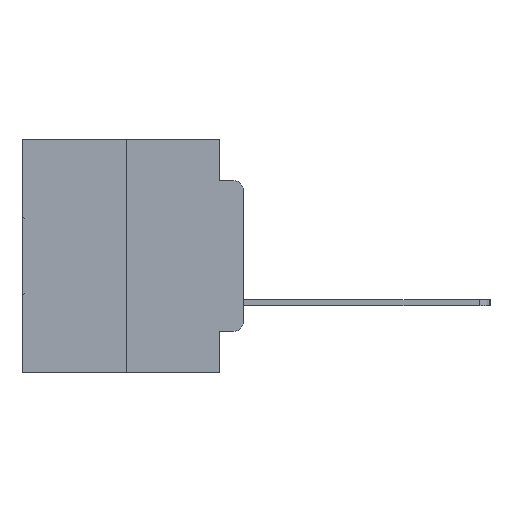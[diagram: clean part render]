
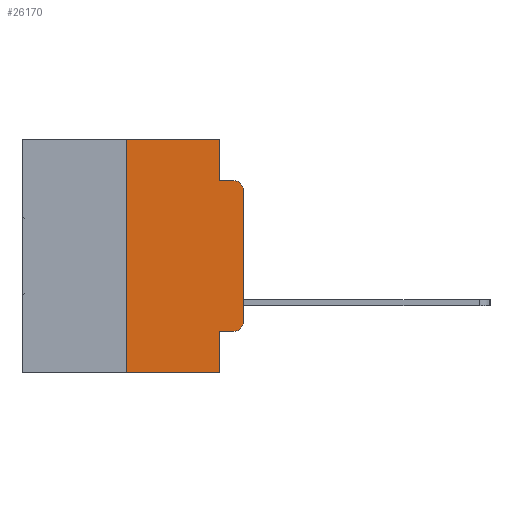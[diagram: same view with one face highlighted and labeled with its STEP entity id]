
A CAD part, left-side view. The second image highlights one B-rep face of the part: STEP entity #26170.
In plain terms, the highlighted planar face has unit normal (-1, 0, 0).
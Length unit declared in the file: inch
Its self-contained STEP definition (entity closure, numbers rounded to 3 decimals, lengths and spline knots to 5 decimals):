
#897 = AXIS2_PLACEMENT_3D ( 'NONE', #19850, #13095, #28838 ) ;
#1126 = CARTESIAN_POINT ( 'NONE',  ( 0., 0.051, 0. ) ) ;
#2217 = VECTOR ( 'NONE', #8518, 39.37008 ) ;
#2575 = ORIENTED_EDGE ( 'NONE', *, *, #15115, .T. ) ;
#2579 = DIRECTION ( 'NONE',  ( 0., -1., 0. ) ) ;
#3057 = ORIENTED_EDGE ( 'NONE', *, *, #19452, .F. ) ;
#3365 = EDGE_CURVE ( 'NONE', #27262, #29498, #6270, .T. ) ;
#3592 = DIRECTION ( 'NONE',  ( 0., 0., -1. ) ) ;
#3678 = ORIENTED_EDGE ( 'NONE', *, *, #18886, .T. ) ;
#3823 = ORIENTED_EDGE ( 'NONE', *, *, #13193, .T. ) ;
#4357 = LINE ( 'NONE', #19909, #27951 ) ;
#4920 = EDGE_CURVE ( 'NONE', #29498, #24131, #13517, .T. ) ;
#4981 = DIRECTION ( 'NONE',  ( 0., -1., 0. ) ) ;
#5535 = ORIENTED_EDGE ( 'NONE', *, *, #6493, .T. ) ;
#5583 = CARTESIAN_POINT ( 'NONE',  ( 0., 0.051, 0. ) ) ;
#6233 = ORIENTED_EDGE ( 'NONE', *, *, #4920, .F. ) ;
#6270 = LINE ( 'NONE', #1126, #23201 ) ;
#6363 = ORIENTED_EDGE ( 'NONE', *, *, #3365, .F. ) ;
#6493 = EDGE_CURVE ( 'NONE', #21890, #24131, #8255, .T. ) ;
#6508 = ORIENTED_EDGE ( 'NONE', *, *, #21362, .F. ) ;
#6709 = ORIENTED_EDGE ( 'NONE', *, *, #28440, .F. ) ;
#8132 = LINE ( 'NONE', #12979, #12904 ) ;
#8255 = CIRCLE ( 'NONE', #26831, 0.02 ) ;
#8440 = LINE ( 'NONE', #13153, #2217 ) ;
#8518 = DIRECTION ( 'NONE',  ( 0., 0., 1. ) ) ;
#8537 = VERTEX_POINT ( 'NONE', #17197 ) ;
#9056 = VERTEX_POINT ( 'NONE', #28308 ) ;
#9466 = CARTESIAN_POINT ( 'NONE',  ( 0., 0.473, 0. ) ) ;
#9485 = DIRECTION ( 'NONE',  ( -1., 0., 0. ) ) ;
#9794 = CARTESIAN_POINT ( 'NONE',  ( 0., 0.02, -0.1085 ) ) ;
#10277 = DIRECTION ( 'NONE',  ( 0., 0., -1. ) ) ;
#10741 = PLANE ( 'NONE',  #897 ) ;
#10845 = VERTEX_POINT ( 'NONE', #26369 ) ;
#12164 = DIRECTION ( 'NONE',  ( 0., 0., -1. ) ) ;
#12477 = CARTESIAN_POINT ( 'NONE',  ( 0., 0.25, 0. ) ) ;
#12703 = LINE ( 'NONE', #5583, #24085 ) ;
#12904 = VECTOR ( 'NONE', #17611, 39.37008 ) ;
#12979 = CARTESIAN_POINT ( 'NONE',  ( 0., 0.473, -0.5 ) ) ;
#13095 = DIRECTION ( 'NONE',  ( 1., 0., 0. ) ) ;
#13153 = CARTESIAN_POINT ( 'NONE',  ( 0., 0., 0. ) ) ;
#13193 = EDGE_CURVE ( 'NONE', #23762, #21890, #8440, .T. ) ;
#13248 = CARTESIAN_POINT ( 'NONE',  ( 0., 0.051, -0.4115 ) ) ;
#13517 = LINE ( 'NONE', #25501, #18858 ) ;
#13674 = VECTOR ( 'NONE', #4981, 39.37008 ) ;
#13866 = EDGE_LOOP ( 'NONE', ( #3823, #5535, #6233, #6363, #6508, #6709, #3678, #3057, #2575, #15732 ) ) ;
#13877 = CARTESIAN_POINT ( 'NONE',  ( 0., 0.25, 0. ) ) ;
#14156 = EDGE_CURVE ( 'NONE', #9056, #23762, #28999, .T. ) ;
#14174 = CARTESIAN_POINT ( 'NONE',  ( 0., 0., -0.1085 ) ) ;
#15115 = EDGE_CURVE ( 'NONE', #22293, #9056, #4357, .T. ) ;
#15732 = ORIENTED_EDGE ( 'NONE', *, *, #14156, .T. ) ;
#15946 = CARTESIAN_POINT ( 'NONE',  ( 0., 0.051, -0.0885 ) ) ;
#16163 = DIRECTION ( 'NONE',  ( 0., 0., 1. ) ) ;
#16355 = CARTESIAN_POINT ( 'NONE',  ( 0., 0., -0.3915 ) ) ;
#17197 = CARTESIAN_POINT ( 'NONE',  ( 0., 0.25, -0.5 ) ) ;
#17611 = DIRECTION ( 'NONE',  ( 0., -1., 0. ) ) ;
#17667 = DIRECTION ( 'NONE',  ( 0., -1., 0. ) ) ;
#18858 = VECTOR ( 'NONE', #2579, 39.37008 ) ;
#18886 = EDGE_CURVE ( 'NONE', #8537, #10845, #8132, .T. ) ;
#19205 = CARTESIAN_POINT ( 'NONE',  ( 0., 0.051, 0. ) ) ;
#19356 = FACE_OUTER_BOUND ( 'NONE', #13866, .T. ) ;
#19452 = EDGE_CURVE ( 'NONE', #22293, #10845, #12703, .T. ) ;
#19850 = CARTESIAN_POINT ( 'NONE',  ( 0., 0.473, 0. ) ) ;
#19909 = CARTESIAN_POINT ( 'NONE',  ( 0., 0.051, -0.4115 ) ) ;
#20413 = LINE ( 'NONE', #9466, #13674 ) ;
#21362 = EDGE_CURVE ( 'NONE', #29782, #27262, #20413, .T. ) ;
#21610 = AXIS2_PLACEMENT_3D ( 'NONE', #23237, #9485, #25457 ) ;
#21890 = VERTEX_POINT ( 'NONE', #14174 ) ;
#22293 = VERTEX_POINT ( 'NONE', #13248 ) ;
#22432 = VECTOR ( 'NONE', #16163, 39.37008 ) ;
#23201 = VECTOR ( 'NONE', #3592, 39.37008 ) ;
#23237 = CARTESIAN_POINT ( 'NONE',  ( 0., 0.02, -0.3915 ) ) ;
#23762 = VERTEX_POINT ( 'NONE', #16355 ) ;
#24085 = VECTOR ( 'NONE', #10277, 39.37008 ) ;
#24131 = VERTEX_POINT ( 'NONE', #24325 ) ;
#24325 = CARTESIAN_POINT ( 'NONE',  ( 0., 0.02, -0.0885 ) ) ;
#25457 = DIRECTION ( 'NONE',  ( 0., 0., -1. ) ) ;
#25501 = CARTESIAN_POINT ( 'NONE',  ( 0., 0.051, -0.0885 ) ) ;
#25750 = DIRECTION ( 'NONE',  ( -1., 0., 0. ) ) ;
#26170 = ADVANCED_FACE ( 'NONE', ( #19356 ), #10741, .F. ) ;
#26369 = CARTESIAN_POINT ( 'NONE',  ( 0., 0.051, -0.5 ) ) ;
#26831 = AXIS2_PLACEMENT_3D ( 'NONE', #9794, #25750, #12164 ) ;
#27262 = VERTEX_POINT ( 'NONE', #19205 ) ;
#27951 = VECTOR ( 'NONE', #17667, 39.37008 ) ;
#28306 = LINE ( 'NONE', #13877, #22432 ) ;
#28308 = CARTESIAN_POINT ( 'NONE',  ( 0., 0.02, -0.4115 ) ) ;
#28440 = EDGE_CURVE ( 'NONE', #8537, #29782, #28306, .T. ) ;
#28838 = DIRECTION ( 'NONE',  ( 0., 0., -1. ) ) ;
#28999 = CIRCLE ( 'NONE', #21610, 0.02 ) ;
#29498 = VERTEX_POINT ( 'NONE', #15946 ) ;
#29782 = VERTEX_POINT ( 'NONE', #12477 ) ;
